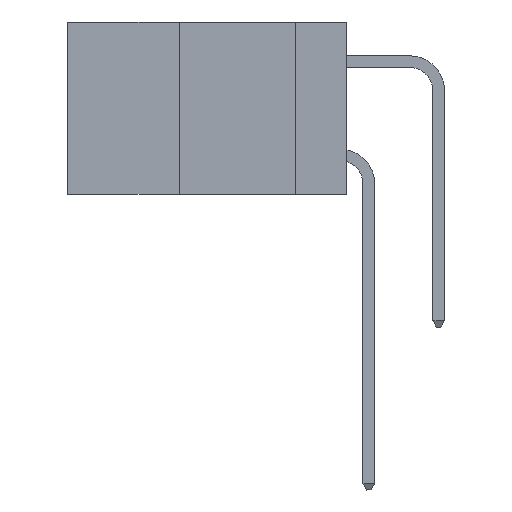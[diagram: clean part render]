
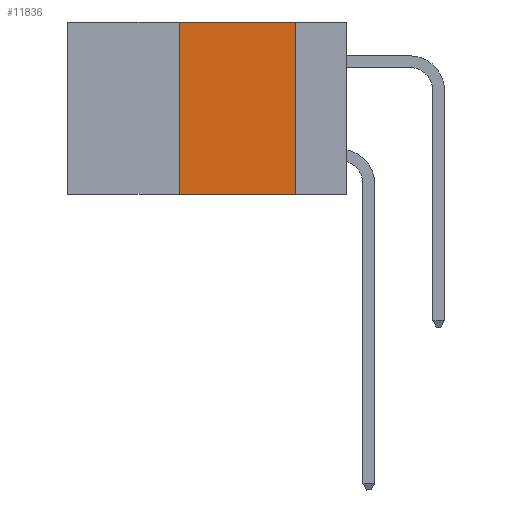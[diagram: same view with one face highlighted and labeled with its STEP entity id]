
A CAD part, left-side view. The second image highlights one B-rep face of the part: STEP entity #11836.
In plain terms, the highlighted planar face has unit normal (-1, 0, 0).
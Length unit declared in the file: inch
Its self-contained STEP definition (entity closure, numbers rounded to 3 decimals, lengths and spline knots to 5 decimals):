
#387 = VERTEX_POINT ( 'NONE', #12632 ) ;
#479 = VERTEX_POINT ( 'NONE', #5271 ) ;
#522 = ORIENTED_EDGE ( 'NONE', *, *, #5643, .F. ) ;
#766 = LINE ( 'NONE', #1927, #10031 ) ;
#949 = CARTESIAN_POINT ( 'NONE',  ( 0., 0.11, -0.37 ) ) ;
#1463 = ORIENTED_EDGE ( 'NONE', *, *, #3298, .F. ) ;
#1927 = CARTESIAN_POINT ( 'NONE',  ( 0., 0.11, 0. ) ) ;
#1950 = VERTEX_POINT ( 'NONE', #10693 ) ;
#1979 = LINE ( 'NONE', #7772, #8538 ) ;
#2056 = CARTESIAN_POINT ( 'NONE',  ( 0., 0.6, -0.37 ) ) ;
#2708 = AXIS2_PLACEMENT_3D ( 'NONE', #2887, #9920, #11832 ) ;
#2810 = EDGE_LOOP ( 'NONE', ( #6317, #1463, #522, #13693 ) ) ;
#2887 = CARTESIAN_POINT ( 'NONE',  ( 0., 0.6, 0. ) ) ;
#3298 = EDGE_CURVE ( 'NONE', #479, #387, #1979, .T. ) ;
#3432 = VECTOR ( 'NONE', #4618, 39.37008 ) ;
#4618 = DIRECTION ( 'NONE',  ( 0., 0., 1. ) ) ;
#5271 = CARTESIAN_POINT ( 'NONE',  ( 0., 0.36, 0. ) ) ;
#5626 = LINE ( 'NONE', #12327, #3432 ) ;
#5643 = EDGE_CURVE ( 'NONE', #1950, #479, #5626, .T. ) ;
#6317 = ORIENTED_EDGE ( 'NONE', *, *, #8890, .F. ) ;
#6359 = DIRECTION ( 'NONE',  ( 0., 0., -1. ) ) ;
#7772 = CARTESIAN_POINT ( 'NONE',  ( 0., 0.6, 0. ) ) ;
#8487 = VECTOR ( 'NONE', #9635, 39.37008 ) ;
#8538 = VECTOR ( 'NONE', #11731, 39.37008 ) ;
#8890 = EDGE_CURVE ( 'NONE', #387, #14348, #766, .T. ) ;
#9635 = DIRECTION ( 'NONE',  ( 0., -1., 0. ) ) ;
#9848 = PLANE ( 'NONE',  #2708 ) ;
#9920 = DIRECTION ( 'NONE',  ( 1., 0., 0. ) ) ;
#10031 = VECTOR ( 'NONE', #6359, 39.37008 ) ;
#10515 = EDGE_CURVE ( 'NONE', #1950, #14348, #11883, .T. ) ;
#10693 = CARTESIAN_POINT ( 'NONE',  ( 0., 0.36, -0.37 ) ) ;
#11071 = FACE_OUTER_BOUND ( 'NONE', #2810, .T. ) ;
#11731 = DIRECTION ( 'NONE',  ( 0., -1., 0. ) ) ;
#11832 = DIRECTION ( 'NONE',  ( 0., 0., -1. ) ) ;
#11836 = ADVANCED_FACE ( 'NONE', ( #11071 ), #9848, .F. ) ;
#11883 = LINE ( 'NONE', #2056, #8487 ) ;
#12327 = CARTESIAN_POINT ( 'NONE',  ( 0., 0.36, 0. ) ) ;
#12632 = CARTESIAN_POINT ( 'NONE',  ( 0., 0.11, 0. ) ) ;
#13693 = ORIENTED_EDGE ( 'NONE', *, *, #10515, .T. ) ;
#14348 = VERTEX_POINT ( 'NONE', #949 ) ;
